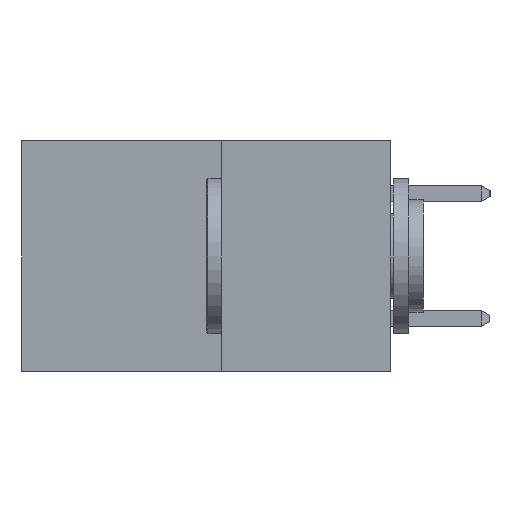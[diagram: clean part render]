
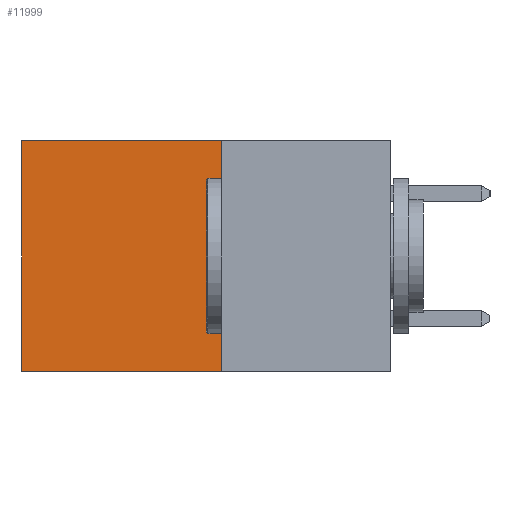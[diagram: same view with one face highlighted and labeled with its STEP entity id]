
A CAD part, left-side view. The second image highlights one B-rep face of the part: STEP entity #11999.
In plain terms, the highlighted planar face has unit normal (-1, 0, 0).
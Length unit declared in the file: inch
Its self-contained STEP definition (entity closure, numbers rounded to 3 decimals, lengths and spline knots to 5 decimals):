
#1134 = VECTOR ( 'NONE', #25690, 39.37008 ) ;
#4792 = LINE ( 'NONE', #5810, #28529 ) ;
#5104 = FACE_OUTER_BOUND ( 'NONE', #9560, .T. ) ;
#5692 = VERTEX_POINT ( 'NONE', #20390 ) ;
#5810 = CARTESIAN_POINT ( 'NONE',  ( 0.277, 0.27, -0.37 ) ) ;
#5837 = EDGE_CURVE ( 'NONE', #5692, #28034, #28112, .T. ) ;
#6699 = CARTESIAN_POINT ( 'NONE',  ( 0.277, 0.59, -0.37 ) ) ;
#7225 = CARTESIAN_POINT ( 'NONE',  ( 0.277, 0.59, -0.37 ) ) ;
#7877 = LINE ( 'NONE', #7225, #1134 ) ;
#8766 = PLANE ( 'NONE',  #12697 ) ;
#9560 = EDGE_LOOP ( 'NONE', ( #19360, #21098, #18488, #10146 ) ) ;
#10146 = ORIENTED_EDGE ( 'NONE', *, *, #18909, .T. ) ;
#11073 = DIRECTION ( 'NONE',  ( 0., 0., -1. ) ) ;
#11838 = VERTEX_POINT ( 'NONE', #28901 ) ;
#11999 = ADVANCED_FACE ( 'NONE', ( #5104 ), #8766, .F. ) ;
#12697 = AXIS2_PLACEMENT_3D ( 'NONE', #17919, #24919, #11073 ) ;
#12823 = EDGE_CURVE ( 'NONE', #12861, #28034, #7877, .T. ) ;
#12861 = VERTEX_POINT ( 'NONE', #21199 ) ;
#15119 = VECTOR ( 'NONE', #28067, 39.37008 ) ;
#17262 = VECTOR ( 'NONE', #18109, 39.37008 ) ;
#17919 = CARTESIAN_POINT ( 'NONE',  ( 0.277, 0.27, -0.37 ) ) ;
#18109 = DIRECTION ( 'NONE',  ( 0., 1., 0. ) ) ;
#18172 = CARTESIAN_POINT ( 'NONE',  ( 0.277, 0.27, -0.37 ) ) ;
#18488 = ORIENTED_EDGE ( 'NONE', *, *, #24273, .F. ) ;
#18909 = EDGE_CURVE ( 'NONE', #11838, #12861, #21281, .T. ) ;
#19360 = ORIENTED_EDGE ( 'NONE', *, *, #12823, .T. ) ;
#19675 = DIRECTION ( 'NONE',  ( 0., 0., -1. ) ) ;
#20390 = CARTESIAN_POINT ( 'NONE',  ( 0.277, 0.27, -0.37 ) ) ;
#21098 = ORIENTED_EDGE ( 'NONE', *, *, #5837, .F. ) ;
#21199 = CARTESIAN_POINT ( 'NONE',  ( 0.277, 0.59, 0. ) ) ;
#21281 = LINE ( 'NONE', #25782, #15119 ) ;
#24273 = EDGE_CURVE ( 'NONE', #11838, #5692, #4792, .T. ) ;
#24919 = DIRECTION ( 'NONE',  ( 1., 0., 0. ) ) ;
#25690 = DIRECTION ( 'NONE',  ( 0., 0., -1. ) ) ;
#25782 = CARTESIAN_POINT ( 'NONE',  ( 0.277, 0.27, 0. ) ) ;
#28034 = VERTEX_POINT ( 'NONE', #6699 ) ;
#28067 = DIRECTION ( 'NONE',  ( 0., 1., 0. ) ) ;
#28112 = LINE ( 'NONE', #18172, #17262 ) ;
#28529 = VECTOR ( 'NONE', #19675, 39.37008 ) ;
#28901 = CARTESIAN_POINT ( 'NONE',  ( 0.277, 0.27, 0. ) ) ;
